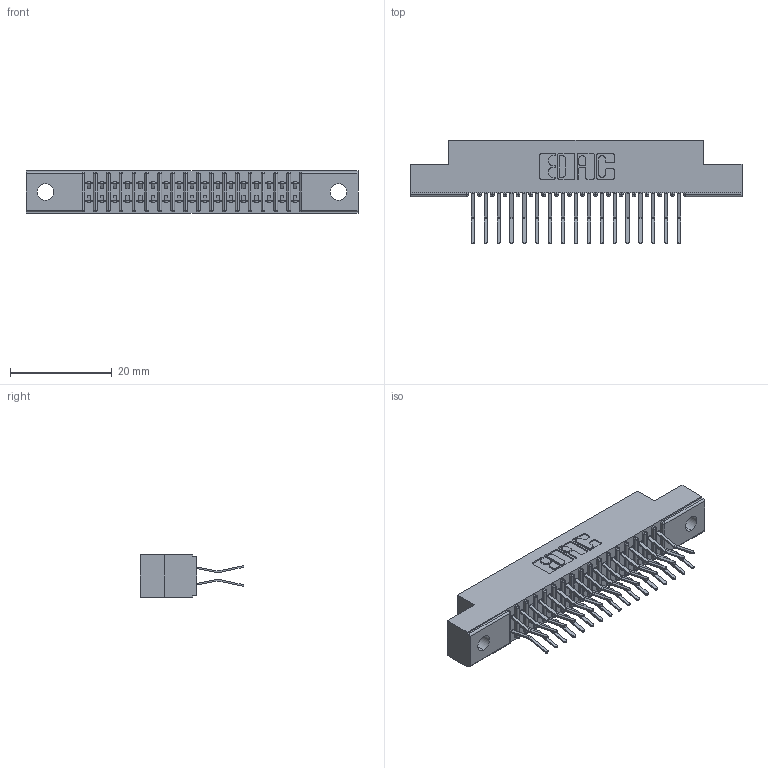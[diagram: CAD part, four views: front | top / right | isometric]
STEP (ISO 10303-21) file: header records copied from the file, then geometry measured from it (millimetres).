
FILE_DESCRIPTION (( 'STEP AP203' ), '1' );
FILE_NAME ('391-034-560-202.STEP', '2018-08-08T23:01:15', ( '' ), ( '' ), 'SwSTEP 2.0', 'SolidWorks 2016', '' );
FILE_SCHEMA (( 'CONFIG_CONTROL_DESIGN' ));
Length unit declared in the file: inch
Products named in the file (3): 341 Part_.128 (3.25) Dia Mounting Holes; 341-292-001_341-292-160; 391-034-560-202
Assembly tree (35 placements, depth 2):
  391-034-560-202
    341 Part_.128 (3.25) Dia Mounting Holes
    341-292-001_341-292-160  x34
Bounding box: 65.41 x 20.37 x 8.38 mm (x, y, z)
Volume: 3730.8 mm3; surface area: 7465.4 mm2
Topology: 35 solids, 35 shells, 2496 faces, 7235 edges, 4694 vertices
Faces by surface type: plane 1428, cylinder 1000, sphere 36, torus 32
Entity records: 24046 total; most frequent: CARTESIAN_POINT 3999, ORIENTED_EDGE 3970, DIRECTION 3903, EDGE_CURVE 1985, LINE 1571, VECTOR 1571, VERTEX_POINT 1262, AXIS2_PLACEMENT_3D 1166
